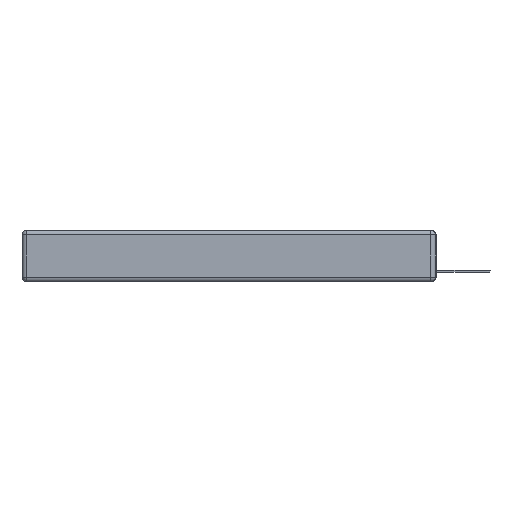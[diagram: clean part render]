
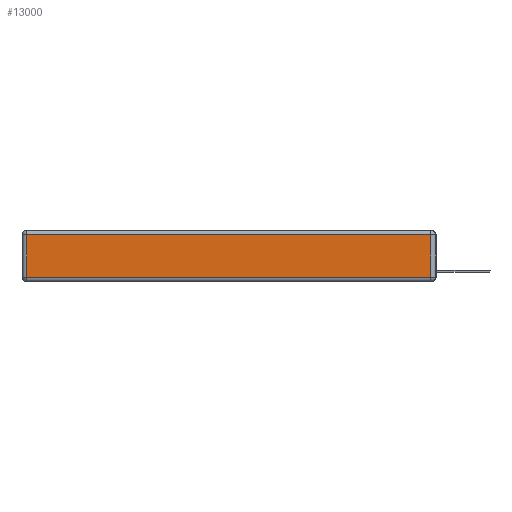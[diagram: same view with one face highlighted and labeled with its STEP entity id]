
A CAD part, left-side view. The second image highlights one B-rep face of the part: STEP entity #13000.
In plain terms, the highlighted planar face has unit normal (-1, 0, 0).
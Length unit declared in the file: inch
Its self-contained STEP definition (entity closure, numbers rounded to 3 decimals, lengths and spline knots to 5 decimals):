
#313 = DIRECTION ( 'NONE',  ( 0., 0., -1. ) ) ;
#905 = AXIS2_PLACEMENT_3D ( 'NONE', #8894, #6999, #12000 ) ;
#2006 = VECTOR ( 'NONE', #8703, 39.37008 ) ;
#3656 = FACE_OUTER_BOUND ( 'NONE', #19572, .T. ) ;
#4459 = ORIENTED_EDGE ( 'NONE', *, *, #19201, .T. ) ;
#5536 = DIRECTION ( 'NONE',  ( 0., 0., 1. ) ) ;
#5612 = PLANE ( 'NONE',  #905 ) ;
#5870 = EDGE_CURVE ( 'NONE', #20265, #15893, #8157, .T. ) ;
#6377 = CARTESIAN_POINT ( 'NONE',  ( 0., 0., -0.313 ) ) ;
#6682 = DIRECTION ( 'NONE',  ( 0., -1., 0. ) ) ;
#6999 = DIRECTION ( 'NONE',  ( -1., 0., 0. ) ) ;
#7113 = ORIENTED_EDGE ( 'NONE', *, *, #13791, .T. ) ;
#8157 = LINE ( 'NONE', #6377, #18727 ) ;
#8493 = CARTESIAN_POINT ( 'NONE',  ( 0., 2.75, -0.03 ) ) ;
#8703 = DIRECTION ( 'NONE',  ( 0., 1., 0. ) ) ;
#8894 = CARTESIAN_POINT ( 'NONE',  ( 0., 0., -0.343 ) ) ;
#9153 = EDGE_CURVE ( 'NONE', #19025, #14727, #12238, .T. ) ;
#9779 = ORIENTED_EDGE ( 'NONE', *, *, #5870, .T. ) ;
#11024 = CARTESIAN_POINT ( 'NONE',  ( 0., 2.72, -0.03 ) ) ;
#11587 = VECTOR ( 'NONE', #5536, 39.37008 ) ;
#12000 = DIRECTION ( 'NONE',  ( 0., 0., 1. ) ) ;
#12139 = LINE ( 'NONE', #20158, #11587 ) ;
#12238 = LINE ( 'NONE', #8493, #2006 ) ;
#13000 = ADVANCED_FACE ( 'NONE', ( #3656 ), #5612, .T. ) ;
#13738 = CARTESIAN_POINT ( 'NONE',  ( 0., 0.03, -0.313 ) ) ;
#13791 = EDGE_CURVE ( 'NONE', #14727, #20265, #15161, .T. ) ;
#14605 = CARTESIAN_POINT ( 'NONE',  ( 0., 0.03, -0.03 ) ) ;
#14727 = VERTEX_POINT ( 'NONE', #11024 ) ;
#15161 = LINE ( 'NONE', #20079, #15573 ) ;
#15573 = VECTOR ( 'NONE', #313, 39.37008 ) ;
#15893 = VERTEX_POINT ( 'NONE', #13738 ) ;
#17053 = ORIENTED_EDGE ( 'NONE', *, *, #9153, .T. ) ;
#17945 = CARTESIAN_POINT ( 'NONE',  ( 0., 2.72, -0.313 ) ) ;
#18727 = VECTOR ( 'NONE', #6682, 39.37008 ) ;
#19025 = VERTEX_POINT ( 'NONE', #14605 ) ;
#19201 = EDGE_CURVE ( 'NONE', #15893, #19025, #12139, .T. ) ;
#19572 = EDGE_LOOP ( 'NONE', ( #9779, #4459, #17053, #7113 ) ) ;
#20079 = CARTESIAN_POINT ( 'NONE',  ( 0., 2.72, -0.343 ) ) ;
#20158 = CARTESIAN_POINT ( 'NONE',  ( 0., 0.03, -0.343 ) ) ;
#20265 = VERTEX_POINT ( 'NONE', #17945 ) ;
